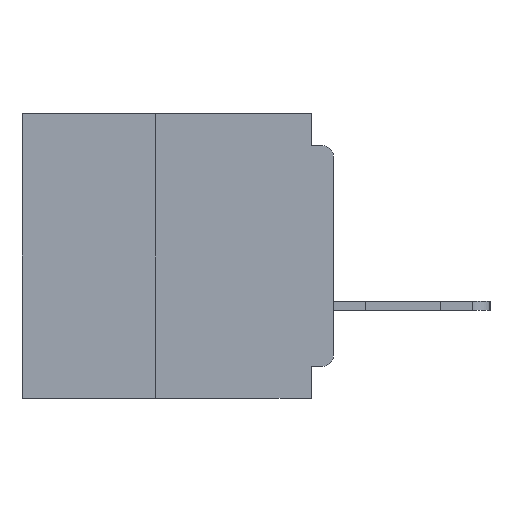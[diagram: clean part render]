
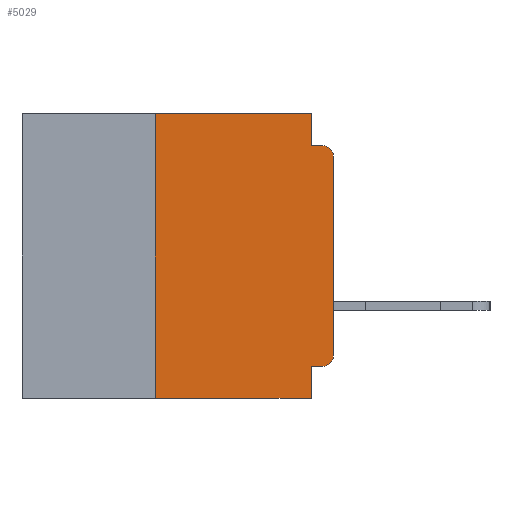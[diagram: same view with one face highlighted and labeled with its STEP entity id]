
A CAD part, left-side view. The second image highlights one B-rep face of the part: STEP entity #5029.
In plain terms, the highlighted planar face has unit normal (-1, 0, 0).
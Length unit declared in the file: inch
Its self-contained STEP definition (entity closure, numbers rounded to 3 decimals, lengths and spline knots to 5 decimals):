
#400 = DIRECTION ( 'NONE',  ( -1., 0., 0. ) ) ;
#770 = VERTEX_POINT ( 'NONE', #14284 ) ;
#2650 = EDGE_CURVE ( 'NONE', #5019, #23827, #31170, .T. ) ;
#3694 = VECTOR ( 'NONE', #24711, 39.37008 ) ;
#4309 = CARTESIAN_POINT ( 'NONE',  ( 0., 0.031, -0.355 ) ) ;
#4984 = VECTOR ( 'NONE', #14413, 39.37008 ) ;
#5019 = VERTEX_POINT ( 'NONE', #29741 ) ;
#5029 = ADVANCED_FACE ( 'NONE', ( #23033 ), #28657, .F. ) ;
#5347 = VERTEX_POINT ( 'NONE', #20962 ) ;
#6164 = VERTEX_POINT ( 'NONE', #4309 ) ;
#6867 = LINE ( 'NONE', #21580, #22726 ) ;
#6880 = AXIS2_PLACEMENT_3D ( 'NONE', #28704, #28384, #28350 ) ;
#7599 = AXIS2_PLACEMENT_3D ( 'NONE', #31016, #30965, #30933 ) ;
#7785 = VECTOR ( 'NONE', #26053, 39.37008 ) ;
#7968 = CIRCLE ( 'NONE', #34583, 0.015 ) ;
#8070 = ORIENTED_EDGE ( 'NONE', *, *, #2650, .T. ) ;
#8234 = CARTESIAN_POINT ( 'NONE',  ( 0., 0.437, -0.4 ) ) ;
#9046 = EDGE_CURVE ( 'NONE', #35180, #40967, #7968, .T. ) ;
#9060 = ORIENTED_EDGE ( 'NONE', *, *, #27102, .F. ) ;
#10422 = EDGE_CURVE ( 'NONE', #23827, #35180, #6867, .T. ) ;
#11194 = LINE ( 'NONE', #19011, #34494 ) ;
#11380 = VECTOR ( 'NONE', #15983, 39.37008 ) ;
#11903 = CARTESIAN_POINT ( 'NONE',  ( 0., 0., -0.34 ) ) ;
#12071 = ORIENTED_EDGE ( 'NONE', *, *, #18544, .F. ) ;
#12764 = ORIENTED_EDGE ( 'NONE', *, *, #10422, .T. ) ;
#13296 = CARTESIAN_POINT ( 'NONE',  ( 0., 0.015, -0.045 ) ) ;
#13309 = CARTESIAN_POINT ( 'NONE',  ( 0., 0., -0.355 ) ) ;
#13467 = LINE ( 'NONE', #20622, #4984 ) ;
#13817 = ORIENTED_EDGE ( 'NONE', *, *, #20680, .T. ) ;
#14284 = CARTESIAN_POINT ( 'NONE',  ( 0., 0.031, -0.4 ) ) ;
#14413 = DIRECTION ( 'NONE',  ( 0., 0., -1. ) ) ;
#15931 = VERTEX_POINT ( 'NONE', #39450 ) ;
#15983 = DIRECTION ( 'NONE',  ( 0., 0., 1. ) ) ;
#17520 = EDGE_CURVE ( 'NONE', #5019, #6164, #34087, .T. ) ;
#17653 = ORIENTED_EDGE ( 'NONE', *, *, #39221, .F. ) ;
#18544 = EDGE_CURVE ( 'NONE', #6164, #770, #11194, .T. ) ;
#19011 = CARTESIAN_POINT ( 'NONE',  ( 0., 0.031, -0.4 ) ) ;
#19550 = CARTESIAN_POINT ( 'NONE',  ( 0., 0.015, -0.06 ) ) ;
#20622 = CARTESIAN_POINT ( 'NONE',  ( 0., 0.031, 0. ) ) ;
#20680 = EDGE_CURVE ( 'NONE', #5347, #770, #29395, .T. ) ;
#20962 = CARTESIAN_POINT ( 'NONE',  ( 0., 0.25, -0.4 ) ) ;
#21517 = CARTESIAN_POINT ( 'NONE',  ( 0., 0., -0.045 ) ) ;
#21535 = VERTEX_POINT ( 'NONE', #37818 ) ;
#21580 = CARTESIAN_POINT ( 'NONE',  ( 0., 0., 0. ) ) ;
#22726 = VECTOR ( 'NONE', #24776, 39.37008 ) ;
#22828 = EDGE_CURVE ( 'NONE', #5347, #29216, #36653, .T. ) ;
#23033 = FACE_OUTER_BOUND ( 'NONE', #28024, .T. ) ;
#23275 = ORIENTED_EDGE ( 'NONE', *, *, #17520, .F. ) ;
#23827 = VERTEX_POINT ( 'NONE', #11903 ) ;
#24139 = CARTESIAN_POINT ( 'NONE',  ( 0., 0., -0.06 ) ) ;
#24711 = DIRECTION ( 'NONE',  ( 0., -1., 0. ) ) ;
#24776 = DIRECTION ( 'NONE',  ( 0., 0., 1. ) ) ;
#25397 = ORIENTED_EDGE ( 'NONE', *, *, #32437, .F. ) ;
#25662 = VECTOR ( 'NONE', #37994, 39.37008 ) ;
#26053 = DIRECTION ( 'NONE',  ( 0., 1., 0. ) ) ;
#27102 = EDGE_CURVE ( 'NONE', #15931, #21535, #13467, .T. ) ;
#28024 = EDGE_LOOP ( 'NONE', ( #12764, #37877, #25397, #9060, #17653, #38503, #13817, #12071, #23275, #8070 ) ) ;
#28350 = DIRECTION ( 'NONE',  ( 0., 0., -1. ) ) ;
#28384 = DIRECTION ( 'NONE',  ( 1., 0., 0. ) ) ;
#28657 = PLANE ( 'NONE',  #6880 ) ;
#28704 = CARTESIAN_POINT ( 'NONE',  ( 0., 0.437, 0. ) ) ;
#29026 = LINE ( 'NONE', #21517, #3694 ) ;
#29216 = VERTEX_POINT ( 'NONE', #32147 ) ;
#29395 = LINE ( 'NONE', #8234, #37806 ) ;
#29741 = CARTESIAN_POINT ( 'NONE',  ( 0., 0.015, -0.355 ) ) ;
#30397 = DIRECTION ( 'NONE',  ( 0., -1., 0. ) ) ;
#30933 = DIRECTION ( 'NONE',  ( 0., 0., -1. ) ) ;
#30965 = DIRECTION ( 'NONE',  ( -1., 0., 0. ) ) ;
#31016 = CARTESIAN_POINT ( 'NONE',  ( 0., 0.015, -0.34 ) ) ;
#31170 = CIRCLE ( 'NONE', #7599, 0.015 ) ;
#32147 = CARTESIAN_POINT ( 'NONE',  ( 0., 0.25, 0. ) ) ;
#32437 = EDGE_CURVE ( 'NONE', #21535, #40967, #29026, .T. ) ;
#34087 = LINE ( 'NONE', #13309, #7785 ) ;
#34101 = LINE ( 'NONE', #41025, #25662 ) ;
#34494 = VECTOR ( 'NONE', #34860, 39.37008 ) ;
#34583 = AXIS2_PLACEMENT_3D ( 'NONE', #19550, #400, #36682 ) ;
#34860 = DIRECTION ( 'NONE',  ( 0., 0., -1. ) ) ;
#35006 = CARTESIAN_POINT ( 'NONE',  ( 0., 0.25, -0.4 ) ) ;
#35180 = VERTEX_POINT ( 'NONE', #24139 ) ;
#36653 = LINE ( 'NONE', #35006, #11380 ) ;
#36682 = DIRECTION ( 'NONE',  ( 0., 0., -1. ) ) ;
#37806 = VECTOR ( 'NONE', #30397, 39.37008 ) ;
#37818 = CARTESIAN_POINT ( 'NONE',  ( 0., 0.031, -0.045 ) ) ;
#37877 = ORIENTED_EDGE ( 'NONE', *, *, #9046, .T. ) ;
#37994 = DIRECTION ( 'NONE',  ( 0., -1., 0. ) ) ;
#38503 = ORIENTED_EDGE ( 'NONE', *, *, #22828, .F. ) ;
#39221 = EDGE_CURVE ( 'NONE', #29216, #15931, #34101, .T. ) ;
#39450 = CARTESIAN_POINT ( 'NONE',  ( 0., 0.031, 0. ) ) ;
#40967 = VERTEX_POINT ( 'NONE', #13296 ) ;
#41025 = CARTESIAN_POINT ( 'NONE',  ( 0., 0.437, 0. ) ) ;
